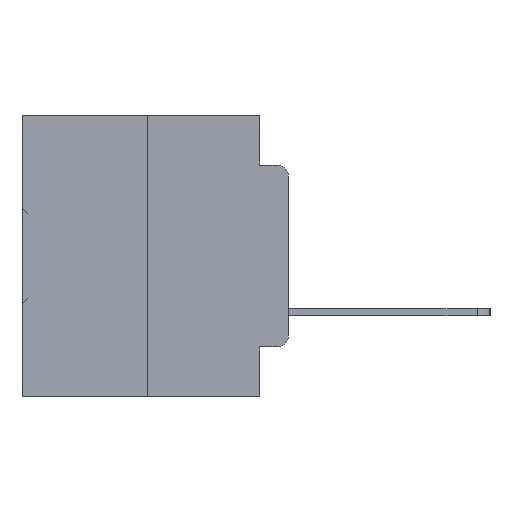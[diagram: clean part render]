
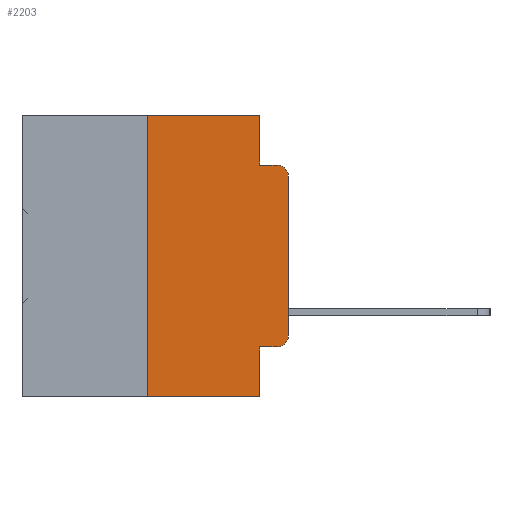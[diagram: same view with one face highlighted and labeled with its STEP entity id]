
A CAD part, left-side view. The second image highlights one B-rep face of the part: STEP entity #2203.
In plain terms, the highlighted planar face has unit normal (-1, 0, 0).
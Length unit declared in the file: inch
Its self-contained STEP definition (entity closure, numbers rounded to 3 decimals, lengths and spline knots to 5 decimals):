
#14 = ORIENTED_EDGE ( 'NONE', *, *, #11786, .T. ) ;
#978 = ORIENTED_EDGE ( 'NONE', *, *, #13829, .T. ) ;
#1636 = CARTESIAN_POINT ( 'NONE',  ( 0., 0.02, -0.1085 ) ) ;
#1646 = DIRECTION ( 'NONE',  ( 0., 0., -1. ) ) ;
#1861 = LINE ( 'NONE', #28294, #16046 ) ;
#2026 = CARTESIAN_POINT ( 'NONE',  ( 0., 0.02, -0.0885 ) ) ;
#2203 = ADVANCED_FACE ( 'NONE', ( #33892 ), #17788, .F. ) ;
#2208 = CARTESIAN_POINT ( 'NONE',  ( 0., 0.051, 0. ) ) ;
#2986 = EDGE_CURVE ( 'NONE', #5600, #32859, #14990, .T. ) ;
#3390 = ORIENTED_EDGE ( 'NONE', *, *, #34220, .F. ) ;
#3824 = CARTESIAN_POINT ( 'NONE',  ( 0., 0.473, 0. ) ) ;
#4085 = VECTOR ( 'NONE', #21239, 39.37008 ) ;
#4631 = DIRECTION ( 'NONE',  ( 0., 0., -1. ) ) ;
#5178 = DIRECTION ( 'NONE',  ( 0., 0., 1. ) ) ;
#5600 = VERTEX_POINT ( 'NONE', #27249 ) ;
#7887 = VECTOR ( 'NONE', #15058, 39.37008 ) ;
#8258 = ORIENTED_EDGE ( 'NONE', *, *, #15835, .T. ) ;
#8262 = VECTOR ( 'NONE', #15654, 39.37008 ) ;
#9643 = CARTESIAN_POINT ( 'NONE',  ( 0., 0., -0.3915 ) ) ;
#9851 = CARTESIAN_POINT ( 'NONE',  ( 0., 0.051, 0. ) ) ;
#10101 = EDGE_CURVE ( 'NONE', #18727, #31262, #33150, .T. ) ;
#10264 = EDGE_LOOP ( 'NONE', ( #8258, #12026, #13419, #22582, #25805, #29690, #14, #3390, #13363, #978 ) ) ;
#11645 = CARTESIAN_POINT ( 'NONE',  ( 0., 0.051, -0.0885 ) ) ;
#11786 = EDGE_CURVE ( 'NONE', #34616, #12589, #15262, .T. ) ;
#12026 = ORIENTED_EDGE ( 'NONE', *, *, #2986, .T. ) ;
#12362 = CARTESIAN_POINT ( 'NONE',  ( 0., 0.473, 0. ) ) ;
#12472 = DIRECTION ( 'NONE',  ( 0., -1., 0. ) ) ;
#12589 = VERTEX_POINT ( 'NONE', #30165 ) ;
#12784 = CIRCLE ( 'NONE', #31690, 0.02 ) ;
#12792 = DIRECTION ( 'NONE',  ( 1., 0., 0. ) ) ;
#13363 = ORIENTED_EDGE ( 'NONE', *, *, #10101, .T. ) ;
#13374 = EDGE_CURVE ( 'NONE', #14924, #32859, #25284, .T. ) ;
#13419 = ORIENTED_EDGE ( 'NONE', *, *, #13374, .F. ) ;
#13639 = EDGE_CURVE ( 'NONE', #21788, #14758, #32756, .T. ) ;
#13829 = EDGE_CURVE ( 'NONE', #31262, #13852, #12784, .T. ) ;
#13852 = VERTEX_POINT ( 'NONE', #9643 ) ;
#14374 = AXIS2_PLACEMENT_3D ( 'NONE', #1636, #21224, #4631 ) ;
#14758 = VERTEX_POINT ( 'NONE', #2208 ) ;
#14924 = VERTEX_POINT ( 'NONE', #19609 ) ;
#14990 = CIRCLE ( 'NONE', #14374, 0.02 ) ;
#15058 = DIRECTION ( 'NONE',  ( 0., -1., 0. ) ) ;
#15169 = DIRECTION ( 'NONE',  ( -1., 0., 0. ) ) ;
#15262 = LINE ( 'NONE', #31154, #7887 ) ;
#15654 = DIRECTION ( 'NONE',  ( 0., 0., 1. ) ) ;
#15835 = EDGE_CURVE ( 'NONE', #13852, #5600, #21944, .T. ) ;
#16046 = VECTOR ( 'NONE', #30932, 39.37008 ) ;
#17788 = PLANE ( 'NONE',  #20648 ) ;
#18088 = VECTOR ( 'NONE', #30477, 39.37008 ) ;
#18372 = CARTESIAN_POINT ( 'NONE',  ( 0., 0., 0. ) ) ;
#18727 = VERTEX_POINT ( 'NONE', #24816 ) ;
#19609 = CARTESIAN_POINT ( 'NONE',  ( 0., 0.051, -0.0885 ) ) ;
#20540 = EDGE_CURVE ( 'NONE', #34616, #21788, #29455, .T. ) ;
#20648 = AXIS2_PLACEMENT_3D ( 'NONE', #12362, #12792, #1646 ) ;
#21224 = DIRECTION ( 'NONE',  ( -1., 0., 0. ) ) ;
#21239 = DIRECTION ( 'NONE',  ( 0., -1., 0. ) ) ;
#21446 = LINE ( 'NONE', #9851, #27796 ) ;
#21788 = VERTEX_POINT ( 'NONE', #26162 ) ;
#21944 = LINE ( 'NONE', #18372, #8262 ) ;
#22582 = ORIENTED_EDGE ( 'NONE', *, *, #35520, .F. ) ;
#24816 = CARTESIAN_POINT ( 'NONE',  ( 0., 0.051, -0.4115 ) ) ;
#25284 = LINE ( 'NONE', #11645, #18088 ) ;
#25805 = ORIENTED_EDGE ( 'NONE', *, *, #13639, .F. ) ;
#26162 = CARTESIAN_POINT ( 'NONE',  ( 0., 0.25, 0. ) ) ;
#26642 = CARTESIAN_POINT ( 'NONE',  ( 0., 0.02, -0.4115 ) ) ;
#27249 = CARTESIAN_POINT ( 'NONE',  ( 0., 0., -0.1085 ) ) ;
#27410 = VECTOR ( 'NONE', #12472, 39.37008 ) ;
#27758 = CARTESIAN_POINT ( 'NONE',  ( 0., 0.25, -0.5 ) ) ;
#27796 = VECTOR ( 'NONE', #28942, 39.37008 ) ;
#28294 = CARTESIAN_POINT ( 'NONE',  ( 0., 0.051, 0. ) ) ;
#28942 = DIRECTION ( 'NONE',  ( 0., 0., -1. ) ) ;
#29455 = LINE ( 'NONE', #29829, #35627 ) ;
#29690 = ORIENTED_EDGE ( 'NONE', *, *, #20540, .F. ) ;
#29829 = CARTESIAN_POINT ( 'NONE',  ( 0., 0.25, 0. ) ) ;
#30165 = CARTESIAN_POINT ( 'NONE',  ( 0., 0.051, -0.5 ) ) ;
#30477 = DIRECTION ( 'NONE',  ( 0., -1., 0. ) ) ;
#30932 = DIRECTION ( 'NONE',  ( 0., 0., -1. ) ) ;
#31154 = CARTESIAN_POINT ( 'NONE',  ( 0., 0.473, -0.5 ) ) ;
#31262 = VERTEX_POINT ( 'NONE', #26642 ) ;
#31264 = CARTESIAN_POINT ( 'NONE',  ( 0., 0.02, -0.3915 ) ) ;
#31690 = AXIS2_PLACEMENT_3D ( 'NONE', #31264, #15169, #33902 ) ;
#31882 = CARTESIAN_POINT ( 'NONE',  ( 0., 0.051, -0.4115 ) ) ;
#32756 = LINE ( 'NONE', #3824, #27410 ) ;
#32859 = VERTEX_POINT ( 'NONE', #2026 ) ;
#33150 = LINE ( 'NONE', #31882, #4085 ) ;
#33892 = FACE_OUTER_BOUND ( 'NONE', #10264, .T. ) ;
#33902 = DIRECTION ( 'NONE',  ( 0., 0., -1. ) ) ;
#34220 = EDGE_CURVE ( 'NONE', #18727, #12589, #21446, .T. ) ;
#34616 = VERTEX_POINT ( 'NONE', #27758 ) ;
#35520 = EDGE_CURVE ( 'NONE', #14758, #14924, #1861, .T. ) ;
#35627 = VECTOR ( 'NONE', #5178, 39.37008 ) ;
